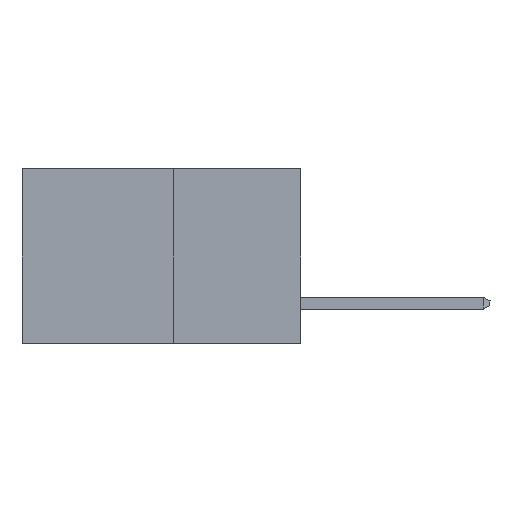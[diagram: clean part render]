
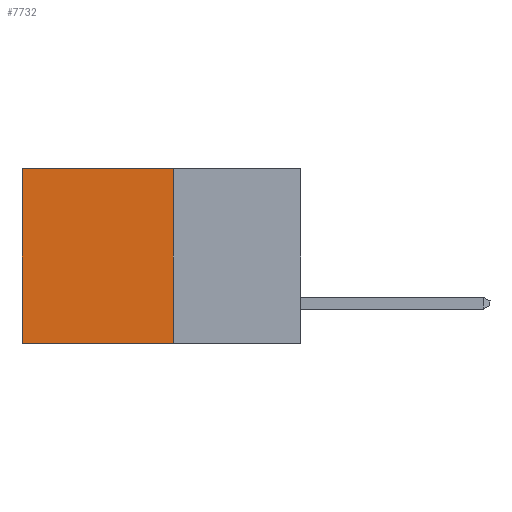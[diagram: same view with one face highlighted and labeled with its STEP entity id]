
A CAD part, left-side view. The second image highlights one B-rep face of the part: STEP entity #7732.
In plain terms, the highlighted planar face has unit normal (-1, 0, 0).
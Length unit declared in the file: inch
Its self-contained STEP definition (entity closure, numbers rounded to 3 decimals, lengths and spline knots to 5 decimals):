
#40 = EDGE_CURVE ( 'NONE', #6086, #11062, #5424, .T. ) ;
#605 = PLANE ( 'NONE',  #4525 ) ;
#958 = VECTOR ( 'NONE', #10172, 39.37008 ) ;
#1175 = VECTOR ( 'NONE', #6413, 39.37008 ) ;
#1177 = DIRECTION ( 'NONE',  ( 0., 0., -1. ) ) ;
#2055 = EDGE_LOOP ( 'NONE', ( #2616, #2600, #2359, #2497 ) ) ;
#2359 = ORIENTED_EDGE ( 'NONE', *, *, #9162, .F. ) ;
#2497 = ORIENTED_EDGE ( 'NONE', *, *, #5256, .T. ) ;
#2600 = ORIENTED_EDGE ( 'NONE', *, *, #3160, .F. ) ;
#2616 = ORIENTED_EDGE ( 'NONE', *, *, #40, .T. ) ;
#3160 = EDGE_CURVE ( 'NONE', #8424, #11062, #4742, .T. ) ;
#3365 = DIRECTION ( 'NONE',  ( 1., 0., 0. ) ) ;
#3895 = CARTESIAN_POINT ( 'NONE',  ( 0.277, 0.27, -0.37 ) ) ;
#4525 = AXIS2_PLACEMENT_3D ( 'NONE', #8445, #3365, #9259 ) ;
#4742 = LINE ( 'NONE', #3895, #7025 ) ;
#4783 = CARTESIAN_POINT ( 'NONE',  ( 0.277, 0.59, -0.37 ) ) ;
#4873 = VECTOR ( 'NONE', #1177, 39.37008 ) ;
#5163 = CARTESIAN_POINT ( 'NONE',  ( 0.277, 0.27, 0. ) ) ;
#5200 = CARTESIAN_POINT ( 'NONE',  ( 0.277, 0.27, -0.37 ) ) ;
#5256 = EDGE_CURVE ( 'NONE', #7046, #6086, #10056, .T. ) ;
#5424 = LINE ( 'NONE', #10518, #4873 ) ;
#6086 = VERTEX_POINT ( 'NONE', #6823 ) ;
#6226 = CARTESIAN_POINT ( 'NONE',  ( 0.277, 0.27, 0. ) ) ;
#6277 = CARTESIAN_POINT ( 'NONE',  ( 0.277, 0.27, -0.37 ) ) ;
#6413 = DIRECTION ( 'NONE',  ( 0., 1., 0. ) ) ;
#6823 = CARTESIAN_POINT ( 'NONE',  ( 0.277, 0.59, 0. ) ) ;
#7025 = VECTOR ( 'NONE', #8648, 39.37008 ) ;
#7046 = VERTEX_POINT ( 'NONE', #5163 ) ;
#7210 = FACE_OUTER_BOUND ( 'NONE', #2055, .T. ) ;
#7732 = ADVANCED_FACE ( 'NONE', ( #7210 ), #605, .F. ) ;
#8193 = LINE ( 'NONE', #5200, #958 ) ;
#8424 = VERTEX_POINT ( 'NONE', #6277 ) ;
#8445 = CARTESIAN_POINT ( 'NONE',  ( 0.277, 0.27, -0.37 ) ) ;
#8648 = DIRECTION ( 'NONE',  ( 0., 1., 0. ) ) ;
#9162 = EDGE_CURVE ( 'NONE', #7046, #8424, #8193, .T. ) ;
#9259 = DIRECTION ( 'NONE',  ( 0., 0., -1. ) ) ;
#10056 = LINE ( 'NONE', #6226, #1175 ) ;
#10172 = DIRECTION ( 'NONE',  ( 0., 0., -1. ) ) ;
#10518 = CARTESIAN_POINT ( 'NONE',  ( 0.277, 0.59, -0.37 ) ) ;
#11062 = VERTEX_POINT ( 'NONE', #4783 ) ;
